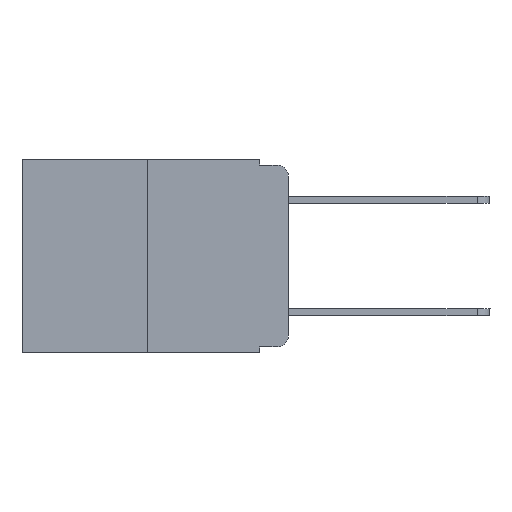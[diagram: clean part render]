
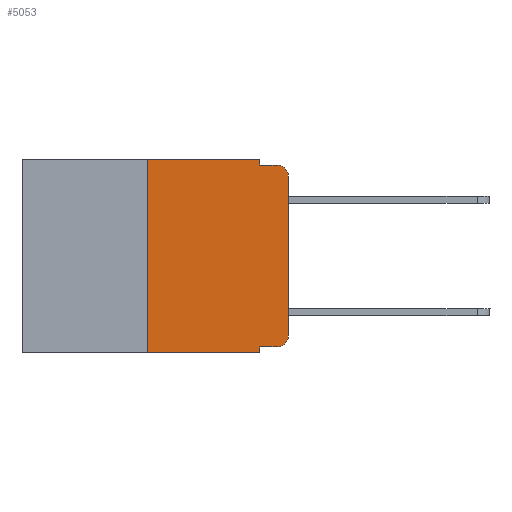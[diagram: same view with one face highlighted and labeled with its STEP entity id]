
A CAD part, left-side view. The second image highlights one B-rep face of the part: STEP entity #5053.
In plain terms, the highlighted planar face has unit normal (-1, 0, 0).
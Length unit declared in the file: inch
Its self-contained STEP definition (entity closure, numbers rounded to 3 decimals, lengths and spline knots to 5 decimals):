
#819 = LINE ( 'NONE', #19855, #20149 ) ;
#861 = CIRCLE ( 'NONE', #15687, 0.02 ) ;
#860 = CARTESIAN_POINT ( 'NONE',  ( 0., 0., -0.03 ) ) ;
#963 = ORIENTED_EDGE ( 'NONE', *, *, #4017, .T. ) ;
#1576 = ORIENTED_EDGE ( 'NONE', *, *, #5720, .F. ) ;
#1690 = CARTESIAN_POINT ( 'NONE',  ( 0., 0.051, -0.343 ) ) ;
#2070 = DIRECTION ( 'NONE',  ( 0., -1., 0. ) ) ;
#2108 = ORIENTED_EDGE ( 'NONE', *, *, #11632, .T. ) ;
#2280 = CARTESIAN_POINT ( 'NONE',  ( 0., 0.051, 0. ) ) ;
#2454 = VECTOR ( 'NONE', #8757, 39.37008 ) ;
#2577 = DIRECTION ( 'NONE',  ( -1., 0., 0. ) ) ;
#2609 = CARTESIAN_POINT ( 'NONE',  ( 0., 0.25, 0. ) ) ;
#2717 = ORIENTED_EDGE ( 'NONE', *, *, #9834, .T. ) ;
#3325 = ORIENTED_EDGE ( 'NONE', *, *, #6322, .F. ) ;
#3426 = EDGE_CURVE ( 'NONE', #15621, #12668, #819, .T. ) ;
#3504 = VERTEX_POINT ( 'NONE', #5793 ) ;
#3570 = EDGE_CURVE ( 'NONE', #12806, #3504, #15513, .T. ) ;
#4017 = EDGE_CURVE ( 'NONE', #8643, #12668, #10755, .T. ) ;
#4585 = VERTEX_POINT ( 'NONE', #1690 ) ;
#4768 = LINE ( 'NONE', #8114, #18111 ) ;
#5051 = PLANE ( 'NONE',  #14698 ) ;
#5053 = ADVANCED_FACE ( 'NONE', ( #19527 ), #5051, .F. ) ;
#5152 = DIRECTION ( 'NONE',  ( 1., 0., 0. ) ) ;
#5383 = AXIS2_PLACEMENT_3D ( 'NONE', #15873, #2577, #6073 ) ;
#5720 = EDGE_CURVE ( 'NONE', #14349, #15621, #18281, .T. ) ;
#5793 = CARTESIAN_POINT ( 'NONE',  ( 0., 0.25, 0. ) ) ;
#5870 = LINE ( 'NONE', #20452, #8931 ) ;
#6073 = DIRECTION ( 'NONE',  ( 0., 0., -1. ) ) ;
#6094 = DIRECTION ( 'NONE',  ( 0., 0., 1. ) ) ;
#6322 = EDGE_CURVE ( 'NONE', #3504, #14349, #5870, .T. ) ;
#6657 = LINE ( 'NONE', #19585, #14806 ) ;
#7201 = CARTESIAN_POINT ( 'NONE',  ( 0., 0.051, -0.333 ) ) ;
#7704 = ORIENTED_EDGE ( 'NONE', *, *, #3426, .F. ) ;
#7927 = CARTESIAN_POINT ( 'NONE',  ( 0., 0.02, -0.313 ) ) ;
#7935 = EDGE_CURVE ( 'NONE', #12806, #4585, #19712, .T. ) ;
#8106 = VERTEX_POINT ( 'NONE', #15467 ) ;
#8114 = CARTESIAN_POINT ( 'NONE',  ( 0., 0., 0. ) ) ;
#8259 = EDGE_CURVE ( 'NONE', #16937, #8106, #861, .T. ) ;
#8643 = VERTEX_POINT ( 'NONE', #860 ) ;
#8707 = DIRECTION ( 'NONE',  ( 0., 0., -1. ) ) ;
#8757 = DIRECTION ( 'NONE',  ( 0., 0., -1. ) ) ;
#8931 = VECTOR ( 'NONE', #18571, 39.37008 ) ;
#9594 = VECTOR ( 'NONE', #2070, 39.37008 ) ;
#9626 = DIRECTION ( 'NONE',  ( -1., 0., 0. ) ) ;
#9722 = VECTOR ( 'NONE', #6094, 39.37008 ) ;
#9834 = EDGE_CURVE ( 'NONE', #8106, #8643, #4768, .T. ) ;
#10324 = VECTOR ( 'NONE', #8707, 39.37008 ) ;
#10755 = CIRCLE ( 'NONE', #5383, 0.02 ) ;
#11393 = CARTESIAN_POINT ( 'NONE',  ( 0., 0.051, -0.01 ) ) ;
#11571 = DIRECTION ( 'NONE',  ( 0., 0., -1. ) ) ;
#11632 = EDGE_CURVE ( 'NONE', #12656, #16937, #6657, .T. ) ;
#12024 = CARTESIAN_POINT ( 'NONE',  ( 0., 0.051, 0. ) ) ;
#12656 = VERTEX_POINT ( 'NONE', #7201 ) ;
#12668 = VERTEX_POINT ( 'NONE', #20329 ) ;
#12806 = VERTEX_POINT ( 'NONE', #19155 ) ;
#14349 = VERTEX_POINT ( 'NONE', #18286 ) ;
#14698 = AXIS2_PLACEMENT_3D ( 'NONE', #19726, #5152, #11571 ) ;
#14806 = VECTOR ( 'NONE', #16158, 39.37008 ) ;
#15467 = CARTESIAN_POINT ( 'NONE',  ( 0., 0., -0.313 ) ) ;
#15513 = LINE ( 'NONE', #2609, #9722 ) ;
#15572 = CARTESIAN_POINT ( 'NONE',  ( 0., 0.02, -0.333 ) ) ;
#15590 = ORIENTED_EDGE ( 'NONE', *, *, #3570, .F. ) ;
#15621 = VERTEX_POINT ( 'NONE', #11393 ) ;
#15687 = AXIS2_PLACEMENT_3D ( 'NONE', #7927, #9626, #19480 ) ;
#15873 = CARTESIAN_POINT ( 'NONE',  ( 0., 0.02, -0.03 ) ) ;
#16158 = DIRECTION ( 'NONE',  ( 0., -1., 0. ) ) ;
#16334 = DIRECTION ( 'NONE',  ( 0., 0., 1. ) ) ;
#16920 = LINE ( 'NONE', #2280, #10324 ) ;
#16937 = VERTEX_POINT ( 'NONE', #15572 ) ;
#16951 = ORIENTED_EDGE ( 'NONE', *, *, #7935, .T. ) ;
#17463 = ORIENTED_EDGE ( 'NONE', *, *, #8259, .T. ) ;
#18002 = CARTESIAN_POINT ( 'NONE',  ( 0., 0.473, -0.343 ) ) ;
#18045 = EDGE_CURVE ( 'NONE', #12656, #4585, #16920, .T. ) ;
#18111 = VECTOR ( 'NONE', #16334, 39.37008 ) ;
#18281 = LINE ( 'NONE', #12024, #2454 ) ;
#18286 = CARTESIAN_POINT ( 'NONE',  ( 0., 0.051, 0. ) ) ;
#18571 = DIRECTION ( 'NONE',  ( 0., -1., 0. ) ) ;
#19155 = CARTESIAN_POINT ( 'NONE',  ( 0., 0.25, -0.343 ) ) ;
#19480 = DIRECTION ( 'NONE',  ( 0., 0., -1. ) ) ;
#19527 = FACE_OUTER_BOUND ( 'NONE', #20873, .T. ) ;
#19585 = CARTESIAN_POINT ( 'NONE',  ( 0., 0.051, -0.333 ) ) ;
#19712 = LINE ( 'NONE', #18002, #9594 ) ;
#19726 = CARTESIAN_POINT ( 'NONE',  ( 0., 0.473, 0. ) ) ;
#19855 = CARTESIAN_POINT ( 'NONE',  ( 0., 0.051, -0.01 ) ) ;
#20149 = VECTOR ( 'NONE', #20278, 39.37008 ) ;
#20278 = DIRECTION ( 'NONE',  ( 0., -1., 0. ) ) ;
#20329 = CARTESIAN_POINT ( 'NONE',  ( 0., 0.02, -0.01 ) ) ;
#20452 = CARTESIAN_POINT ( 'NONE',  ( 0., 0.473, 0. ) ) ;
#20850 = ORIENTED_EDGE ( 'NONE', *, *, #18045, .F. ) ;
#20873 = EDGE_LOOP ( 'NONE', ( #2717, #963, #7704, #1576, #3325, #15590, #16951, #20850, #2108, #17463 ) ) ;
